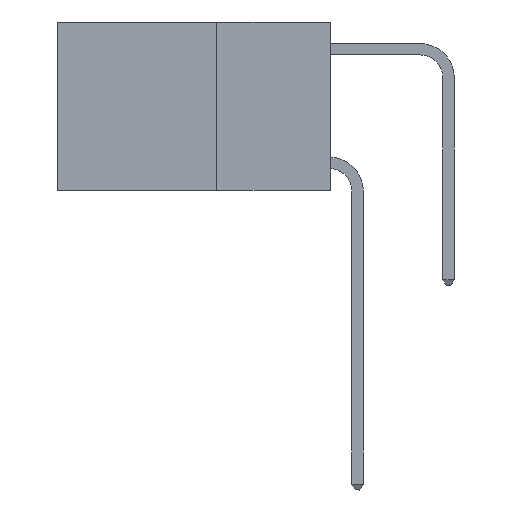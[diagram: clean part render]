
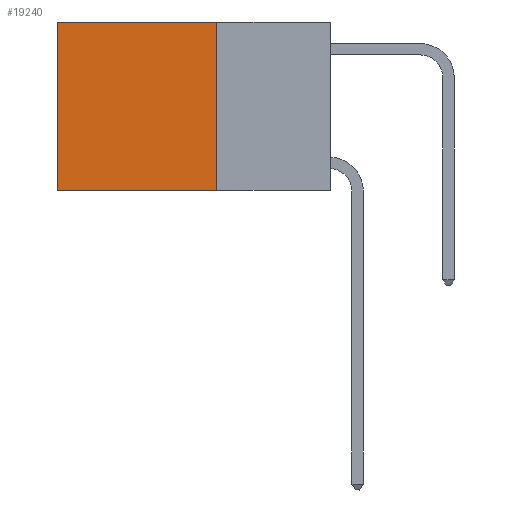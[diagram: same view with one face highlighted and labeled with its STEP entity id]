
A CAD part, left-side view. The second image highlights one B-rep face of the part: STEP entity #19240.
In plain terms, the highlighted planar face has unit normal (-1, 0, 0).
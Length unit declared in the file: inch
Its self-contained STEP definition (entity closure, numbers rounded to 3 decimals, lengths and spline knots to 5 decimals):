
#660 = CARTESIAN_POINT ( 'NONE',  ( 0.2625, 0.25, 0. ) ) ;
#900 = PLANE ( 'NONE',  #5144 ) ;
#1526 = CARTESIAN_POINT ( 'NONE',  ( 0.2625, 0.25, -0.37 ) ) ;
#2583 = VERTEX_POINT ( 'NONE', #15268 ) ;
#2855 = CARTESIAN_POINT ( 'NONE',  ( 0.2625, 0.6, 0. ) ) ;
#4369 = LINE ( 'NONE', #12259, #10864 ) ;
#4835 = FACE_OUTER_BOUND ( 'NONE', #17560, .T. ) ;
#5144 = AXIS2_PLACEMENT_3D ( 'NONE', #660, #8715, #22626 ) ;
#5234 = VERTEX_POINT ( 'NONE', #2855 ) ;
#6016 = VECTOR ( 'NONE', #23980, 39.37008 ) ;
#6225 = EDGE_CURVE ( 'NONE', #20604, #9537, #4369, .T. ) ;
#6307 = ORIENTED_EDGE ( 'NONE', *, *, #6225, .F. ) ;
#7194 = LINE ( 'NONE', #23064, #25166 ) ;
#8596 = LINE ( 'NONE', #16479, #12986 ) ;
#8715 = DIRECTION ( 'NONE',  ( 1., 0., 0. ) ) ;
#9537 = VERTEX_POINT ( 'NONE', #21521 ) ;
#10864 = VECTOR ( 'NONE', #25106, 39.37008 ) ;
#10870 = DIRECTION ( 'NONE',  ( 0., 1., 0. ) ) ;
#12259 = CARTESIAN_POINT ( 'NONE',  ( 0.2625, 0.25, 0. ) ) ;
#12969 = EDGE_CURVE ( 'NONE', #5234, #2583, #7194, .T. ) ;
#12986 = VECTOR ( 'NONE', #10870, 39.37008 ) ;
#14137 = CARTESIAN_POINT ( 'NONE',  ( 0.2625, 0.25, 0. ) ) ;
#15268 = CARTESIAN_POINT ( 'NONE',  ( 0.2625, 0.6, -0.37 ) ) ;
#15927 = LINE ( 'NONE', #1526, #6016 ) ;
#16479 = CARTESIAN_POINT ( 'NONE',  ( 0.2625, 0.25, 0. ) ) ;
#17560 = EDGE_LOOP ( 'NONE', ( #20619, #22138, #6307, #25088 ) ) ;
#19240 = ADVANCED_FACE ( 'NONE', ( #4835 ), #900, .F. ) ;
#19255 = EDGE_CURVE ( 'NONE', #20604, #5234, #8596, .T. ) ;
#19581 = DIRECTION ( 'NONE',  ( 0., 0., -1. ) ) ;
#20604 = VERTEX_POINT ( 'NONE', #14137 ) ;
#20619 = ORIENTED_EDGE ( 'NONE', *, *, #12969, .T. ) ;
#21521 = CARTESIAN_POINT ( 'NONE',  ( 0.2625, 0.25, -0.37 ) ) ;
#22138 = ORIENTED_EDGE ( 'NONE', *, *, #24790, .F. ) ;
#22626 = DIRECTION ( 'NONE',  ( 0., 0., -1. ) ) ;
#23064 = CARTESIAN_POINT ( 'NONE',  ( 0.2625, 0.6, 0. ) ) ;
#23980 = DIRECTION ( 'NONE',  ( 0., 1., 0. ) ) ;
#24790 = EDGE_CURVE ( 'NONE', #9537, #2583, #15927, .T. ) ;
#25088 = ORIENTED_EDGE ( 'NONE', *, *, #19255, .T. ) ;
#25106 = DIRECTION ( 'NONE',  ( 0., 0., -1. ) ) ;
#25166 = VECTOR ( 'NONE', #19581, 39.37008 ) ;
